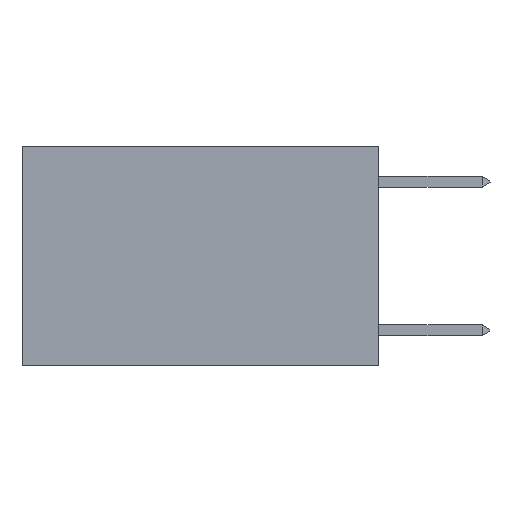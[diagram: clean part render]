
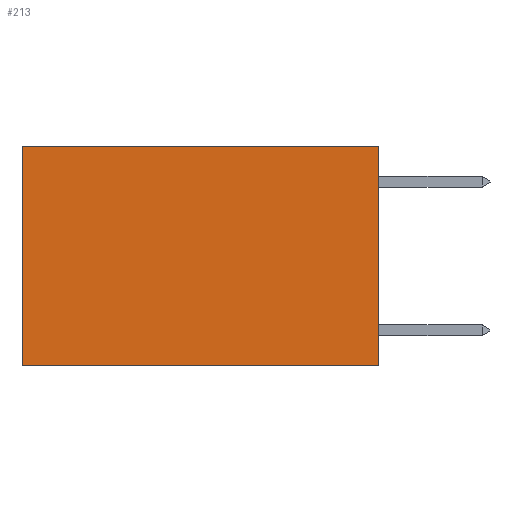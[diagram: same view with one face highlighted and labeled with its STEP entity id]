
A CAD part, left-side view. The second image highlights one B-rep face of the part: STEP entity #213.
In plain terms, the highlighted planar face has unit normal (-1, 0, 0).
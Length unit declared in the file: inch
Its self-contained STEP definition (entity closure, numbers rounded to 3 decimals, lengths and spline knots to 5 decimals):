
#198 = EDGE_CURVE ( 'NONE', #13438, #13021, #4078, .T. ) ;
#213 = ADVANCED_FACE ( 'NONE', ( #9331 ), #9165, .F. ) ;
#333 = DIRECTION ( 'NONE',  ( 0., 1., 0. ) ) ;
#1516 = LINE ( 'NONE', #6284, #10224 ) ;
#1529 = DIRECTION ( 'NONE',  ( 0., 0., -1. ) ) ;
#1815 = CARTESIAN_POINT ( 'NONE',  ( 0.2625, 0., 0. ) ) ;
#2464 = LINE ( 'NONE', #11721, #11121 ) ;
#3341 = CARTESIAN_POINT ( 'NONE',  ( 0.2625, 0.6, 0. ) ) ;
#3633 = EDGE_CURVE ( 'NONE', #14657, #4722, #1516, .T. ) ;
#4078 = LINE ( 'NONE', #11200, #9652 ) ;
#4466 = CARTESIAN_POINT ( 'NONE',  ( 0.2625, 0., -0.37 ) ) ;
#4576 = CARTESIAN_POINT ( 'NONE',  ( 0.2625, 0.6, 0. ) ) ;
#4722 = VERTEX_POINT ( 'NONE', #3341 ) ;
#4826 = DIRECTION ( 'NONE',  ( 1., 0., 0. ) ) ;
#5038 = AXIS2_PLACEMENT_3D ( 'NONE', #8100, #4826, #14813 ) ;
#5624 = VECTOR ( 'NONE', #5714, 39.37008 ) ;
#5714 = DIRECTION ( 'NONE',  ( 0., 0., -1. ) ) ;
#6284 = CARTESIAN_POINT ( 'NONE',  ( 0.2625, 0., 0. ) ) ;
#6940 = DIRECTION ( 'NONE',  ( 0., 1., 0. ) ) ;
#6951 = EDGE_CURVE ( 'NONE', #4722, #13021, #8605, .T. ) ;
#7173 = EDGE_LOOP ( 'NONE', ( #9984, #9904, #9675, #8722 ) ) ;
#8100 = CARTESIAN_POINT ( 'NONE',  ( 0.2625, 0., 0. ) ) ;
#8298 = CARTESIAN_POINT ( 'NONE',  ( 0.2625, 0.6, -0.37 ) ) ;
#8605 = LINE ( 'NONE', #4576, #5624 ) ;
#8722 = ORIENTED_EDGE ( 'NONE', *, *, #3633, .T. ) ;
#8849 = EDGE_CURVE ( 'NONE', #14657, #13438, #2464, .T. ) ;
#9165 = PLANE ( 'NONE',  #5038 ) ;
#9331 = FACE_OUTER_BOUND ( 'NONE', #7173, .T. ) ;
#9652 = VECTOR ( 'NONE', #6940, 39.37008 ) ;
#9675 = ORIENTED_EDGE ( 'NONE', *, *, #8849, .F. ) ;
#9904 = ORIENTED_EDGE ( 'NONE', *, *, #198, .F. ) ;
#9984 = ORIENTED_EDGE ( 'NONE', *, *, #6951, .T. ) ;
#10224 = VECTOR ( 'NONE', #333, 39.37008 ) ;
#11121 = VECTOR ( 'NONE', #1529, 39.37008 ) ;
#11200 = CARTESIAN_POINT ( 'NONE',  ( 0.2625, 0., -0.37 ) ) ;
#11721 = CARTESIAN_POINT ( 'NONE',  ( 0.2625, 0., 0. ) ) ;
#13021 = VERTEX_POINT ( 'NONE', #8298 ) ;
#13438 = VERTEX_POINT ( 'NONE', #4466 ) ;
#14657 = VERTEX_POINT ( 'NONE', #1815 ) ;
#14813 = DIRECTION ( 'NONE',  ( 0., 0., -1. ) ) ;
